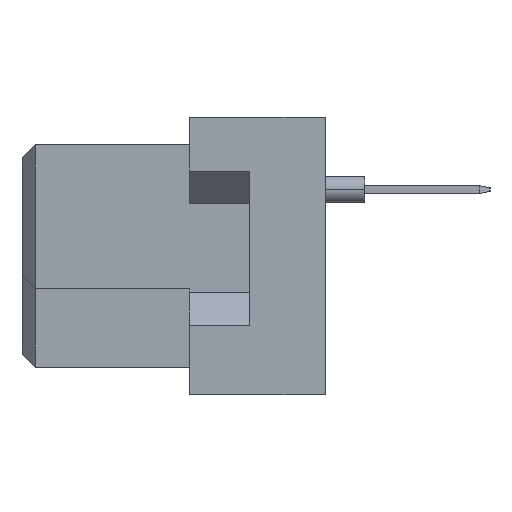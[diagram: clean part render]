
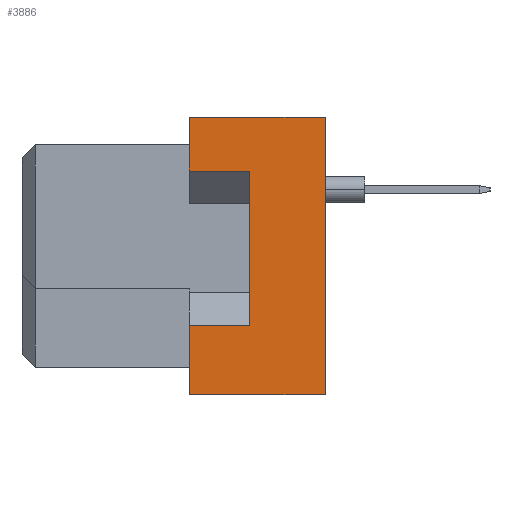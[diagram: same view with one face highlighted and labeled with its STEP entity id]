
A CAD part, left-side view. The second image highlights one B-rep face of the part: STEP entity #3886.
In plain terms, the highlighted planar face has unit normal (-1, 0, 0).
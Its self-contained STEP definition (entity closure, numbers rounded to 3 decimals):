
#604 = VECTOR ( 'NONE', #1124, 1000. ) ;
#1083 = CARTESIAN_POINT ( 'NONE',  ( -27.5, -11.6, 5.3 ) ) ;
#1124 = DIRECTION ( 'NONE',  ( 0., 0., 1. ) ) ;
#1402 = EDGE_CURVE ( 'NONE', #9674, #10996, #19021, .T. ) ;
#1510 = CARTESIAN_POINT ( 'NONE',  ( -27.5, -8.7, -2.65 ) ) ;
#2586 = VECTOR ( 'NONE', #11032, 1000. ) ;
#2791 = CARTESIAN_POINT ( 'NONE',  ( -27.5, -6.4, -5.3 ) ) ;
#3157 = EDGE_CURVE ( 'NONE', #9176, #18950, #10565, .T. ) ;
#3158 = CARTESIAN_POINT ( 'NONE',  ( -27.5, -6.4, -5.3 ) ) ;
#3648 = DIRECTION ( 'NONE',  ( 0., 1., 0. ) ) ;
#3675 = LINE ( 'NONE', #11145, #15262 ) ;
#3886 = ADVANCED_FACE ( 'NONE', ( #18481 ), #6397, .T. ) ;
#4233 = CARTESIAN_POINT ( 'NONE',  ( -27.5, -6.4, 5.3 ) ) ;
#6270 = LINE ( 'NONE', #2791, #17928 ) ;
#6295 = CARTESIAN_POINT ( 'NONE',  ( -27.5, -11.6, 5.3 ) ) ;
#6397 = PLANE ( 'NONE',  #16606 ) ;
#6944 = CARTESIAN_POINT ( 'NONE',  ( -27.5, -11.6, 5.3 ) ) ;
#6964 = CARTESIAN_POINT ( 'NONE',  ( -27.5, -8.7, 3.25 ) ) ;
#7237 = ORIENTED_EDGE ( 'NONE', *, *, #3157, .F. ) ;
#7289 = ORIENTED_EDGE ( 'NONE', *, *, #19285, .F. ) ;
#8629 = ORIENTED_EDGE ( 'NONE', *, *, #12768, .T. ) ;
#9137 = CARTESIAN_POINT ( 'NONE',  ( -27.5, -8.7, 3.25 ) ) ;
#9176 = VERTEX_POINT ( 'NONE', #6964 ) ;
#9578 = VECTOR ( 'NONE', #20196, 1000. ) ;
#9674 = VERTEX_POINT ( 'NONE', #12461 ) ;
#10565 = LINE ( 'NONE', #9137, #9578 ) ;
#10864 = ORIENTED_EDGE ( 'NONE', *, *, #18153, .F. ) ;
#10890 = EDGE_LOOP ( 'NONE', ( #17859, #14767, #10864, #17128, #8629, #7289, #7237, #19764 ) ) ;
#10996 = VERTEX_POINT ( 'NONE', #14510 ) ;
#11002 = DIRECTION ( 'NONE',  ( 0., 0., 1. ) ) ;
#11032 = DIRECTION ( 'NONE',  ( 0., 0., 1. ) ) ;
#11145 = CARTESIAN_POINT ( 'NONE',  ( -27.5, -11.6, -5.3 ) ) ;
#11523 = CARTESIAN_POINT ( 'NONE',  ( -27.5, -8.7, -2.65 ) ) ;
#12188 = CARTESIAN_POINT ( 'NONE',  ( -27.5, -11.6, -5.3 ) ) ;
#12457 = LINE ( 'NONE', #1510, #18221 ) ;
#12461 = CARTESIAN_POINT ( 'NONE',  ( -27.5, -6.4, -5.3 ) ) ;
#12768 = EDGE_CURVE ( 'NONE', #13984, #14298, #13549, .T. ) ;
#13549 = LINE ( 'NONE', #1083, #19850 ) ;
#13984 = VERTEX_POINT ( 'NONE', #6944 ) ;
#14298 = VERTEX_POINT ( 'NONE', #4233 ) ;
#14510 = CARTESIAN_POINT ( 'NONE',  ( -27.5, -6.4, -2.65 ) ) ;
#14767 = ORIENTED_EDGE ( 'NONE', *, *, #1402, .F. ) ;
#15173 = DIRECTION ( 'NONE',  ( 0., 0., 1. ) ) ;
#15262 = VECTOR ( 'NONE', #19230, 1000. ) ;
#15602 = CARTESIAN_POINT ( 'NONE',  ( -27.5, -6.4, 3.25 ) ) ;
#15717 = EDGE_CURVE ( 'NONE', #18182, #10996, #19402, .T. ) ;
#16237 = VECTOR ( 'NONE', #3648, 1000. ) ;
#16408 = VERTEX_POINT ( 'NONE', #12188 ) ;
#16606 = AXIS2_PLACEMENT_3D ( 'NONE', #6295, #20010, #11002 ) ;
#16669 = CARTESIAN_POINT ( 'NONE',  ( -27.5, -8.7, -2.65 ) ) ;
#16693 = EDGE_CURVE ( 'NONE', #16408, #13984, #19452, .T. ) ;
#17128 = ORIENTED_EDGE ( 'NONE', *, *, #16693, .T. ) ;
#17859 = ORIENTED_EDGE ( 'NONE', *, *, #15717, .T. ) ;
#17928 = VECTOR ( 'NONE', #15173, 1000. ) ;
#18153 = EDGE_CURVE ( 'NONE', #16408, #9674, #3675, .T. ) ;
#18175 = DIRECTION ( 'NONE',  ( 0., 1., 0. ) ) ;
#18182 = VERTEX_POINT ( 'NONE', #16669 ) ;
#18221 = VECTOR ( 'NONE', #18499, 1000. ) ;
#18363 = EDGE_CURVE ( 'NONE', #18182, #9176, #12457, .T. ) ;
#18481 = FACE_OUTER_BOUND ( 'NONE', #10890, .T. ) ;
#18499 = DIRECTION ( 'NONE',  ( 0., 0., 1. ) ) ;
#18950 = VERTEX_POINT ( 'NONE', #15602 ) ;
#19021 = LINE ( 'NONE', #3158, #2586 ) ;
#19230 = DIRECTION ( 'NONE',  ( 0., 1., 0. ) ) ;
#19285 = EDGE_CURVE ( 'NONE', #18950, #14298, #6270, .T. ) ;
#19402 = LINE ( 'NONE', #11523, #16237 ) ;
#19452 = LINE ( 'NONE', #19652, #604 ) ;
#19652 = CARTESIAN_POINT ( 'NONE',  ( -27.5, -11.6, 5.3 ) ) ;
#19764 = ORIENTED_EDGE ( 'NONE', *, *, #18363, .F. ) ;
#19850 = VECTOR ( 'NONE', #18175, 1000. ) ;
#20010 = DIRECTION ( 'NONE',  ( -1., 0., 0. ) ) ;
#20196 = DIRECTION ( 'NONE',  ( 0., 1., 0. ) ) ;
